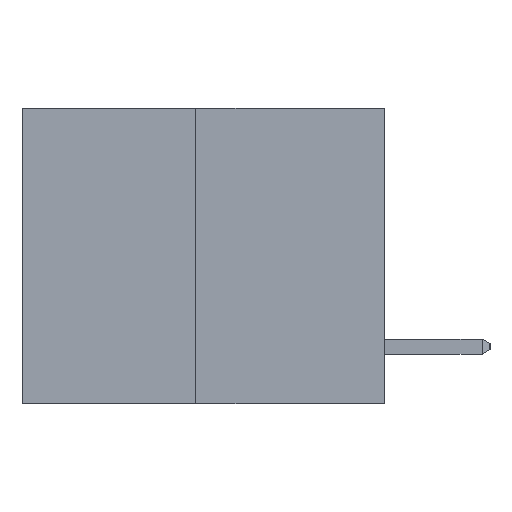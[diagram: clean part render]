
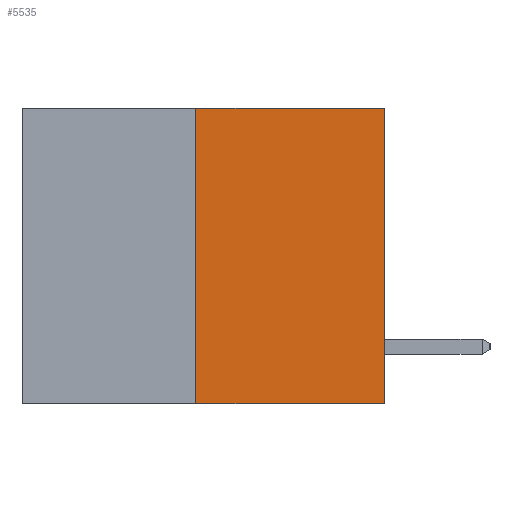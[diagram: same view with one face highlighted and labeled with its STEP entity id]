
A CAD part, left-side view. The second image highlights one B-rep face of the part: STEP entity #5535.
In plain terms, the highlighted planar face has unit normal (-1, 0, 0).
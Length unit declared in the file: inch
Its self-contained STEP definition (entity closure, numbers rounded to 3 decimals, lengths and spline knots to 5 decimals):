
#1239 = VECTOR ( 'NONE', #23806, 39.37008 ) ;
#2676 = LINE ( 'NONE', #8061, #13259 ) ;
#2802 = FACE_OUTER_BOUND ( 'NONE', #21119, .T. ) ;
#3048 = VECTOR ( 'NONE', #9664, 39.37008 ) ;
#5535 = ADVANCED_FACE ( 'NONE', ( #2802 ), #6779, .F. ) ;
#6779 = PLANE ( 'NONE',  #25877 ) ;
#6813 = VERTEX_POINT ( 'NONE', #10971 ) ;
#8061 = CARTESIAN_POINT ( 'NONE',  ( 0., 0.312, -0.49 ) ) ;
#8406 = ORIENTED_EDGE ( 'NONE', *, *, #10488, .F. ) ;
#9664 = DIRECTION ( 'NONE',  ( 0., 0., 1. ) ) ;
#9694 = VERTEX_POINT ( 'NONE', #11811 ) ;
#10488 = EDGE_CURVE ( 'NONE', #14974, #6813, #2676, .T. ) ;
#10971 = CARTESIAN_POINT ( 'NONE',  ( 0., 0.312, 0. ) ) ;
#11177 = ORIENTED_EDGE ( 'NONE', *, *, #26456, .T. ) ;
#11811 = CARTESIAN_POINT ( 'NONE',  ( 0., 0., -0.49 ) ) ;
#11874 = DIRECTION ( 'NONE',  ( 0., -1., 0. ) ) ;
#13257 = ORIENTED_EDGE ( 'NONE', *, *, #22558, .T. ) ;
#13259 = VECTOR ( 'NONE', #26218, 39.37008 ) ;
#14919 = VECTOR ( 'NONE', #11874, 39.37008 ) ;
#14974 = VERTEX_POINT ( 'NONE', #18455 ) ;
#17729 = CARTESIAN_POINT ( 'NONE',  ( 0., 0., 0. ) ) ;
#18279 = CARTESIAN_POINT ( 'NONE',  ( 0., 0.6, 0. ) ) ;
#18377 = DIRECTION ( 'NONE',  ( 0., 0., -1. ) ) ;
#18455 = CARTESIAN_POINT ( 'NONE',  ( 0., 0.312, -0.49 ) ) ;
#19599 = CARTESIAN_POINT ( 'NONE',  ( 0., 0.6, 0. ) ) ;
#20643 = VERTEX_POINT ( 'NONE', #17729 ) ;
#20994 = CARTESIAN_POINT ( 'NONE',  ( 0., 0., 0. ) ) ;
#21119 = EDGE_LOOP ( 'NONE', ( #8406, #13257, #11177, #22265 ) ) ;
#21418 = LINE ( 'NONE', #19599, #1239 ) ;
#22265 = ORIENTED_EDGE ( 'NONE', *, *, #28401, .F. ) ;
#22558 = EDGE_CURVE ( 'NONE', #14974, #9694, #26987, .T. ) ;
#22854 = DIRECTION ( 'NONE',  ( 1., 0., 0. ) ) ;
#23806 = DIRECTION ( 'NONE',  ( 0., -1., 0. ) ) ;
#23975 = LINE ( 'NONE', #20994, #3048 ) ;
#25434 = CARTESIAN_POINT ( 'NONE',  ( 0., 0.6, -0.49 ) ) ;
#25877 = AXIS2_PLACEMENT_3D ( 'NONE', #18279, #22854, #18377 ) ;
#26218 = DIRECTION ( 'NONE',  ( 0., 0., 1. ) ) ;
#26456 = EDGE_CURVE ( 'NONE', #9694, #20643, #23975, .T. ) ;
#26987 = LINE ( 'NONE', #25434, #14919 ) ;
#28401 = EDGE_CURVE ( 'NONE', #6813, #20643, #21418, .T. ) ;
